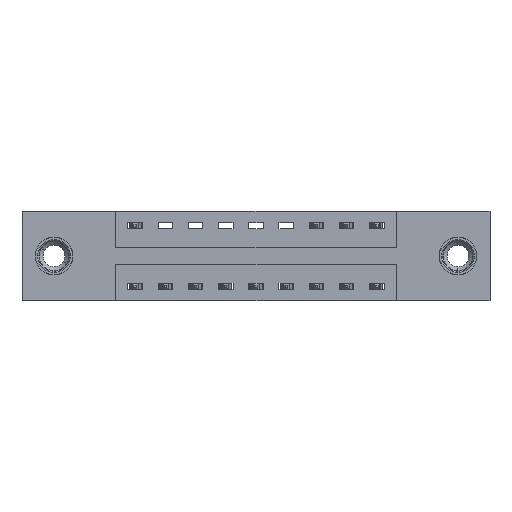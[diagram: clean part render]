
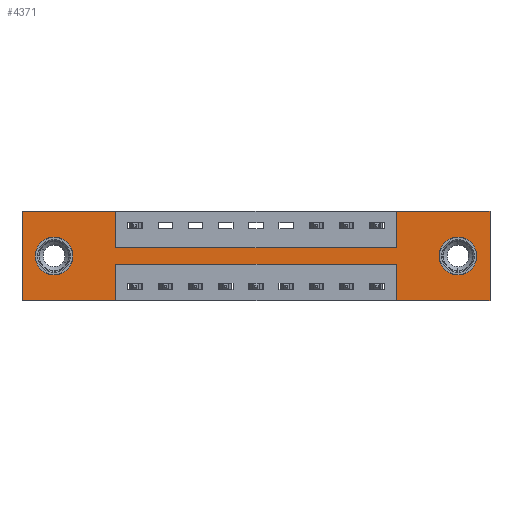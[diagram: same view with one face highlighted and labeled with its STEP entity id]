
A CAD part, front view. The second image highlights one B-rep face of the part: STEP entity #4371.
In plain terms, the highlighted planar face has unit normal (0, -1, 0).
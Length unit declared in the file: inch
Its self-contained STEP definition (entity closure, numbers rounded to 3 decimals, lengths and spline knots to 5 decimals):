
#75 = LINE ( 'NONE', #1002, #4664 ) ;
#83 = ORIENTED_EDGE ( 'NONE', *, *, #7281, .T. ) ;
#263 = DIRECTION ( 'NONE',  ( 0., 0., -1. ) ) ;
#331 = EDGE_CURVE ( 'NONE', #4508, #7372, #1394, .T. ) ;
#455 = EDGE_CURVE ( 'NONE', #640, #3458, #11091, .T. ) ;
#507 = LINE ( 'NONE', #1599, #2647 ) ;
#540 = CARTESIAN_POINT ( 'NONE',  ( 1.935, 0., 0. ) ) ;
#574 = LINE ( 'NONE', #8407, #2717 ) ;
#582 = VECTOR ( 'NONE', #7790, 39.37008 ) ;
#640 = VERTEX_POINT ( 'NONE', #8382 ) ;
#644 = DIRECTION ( 'NONE',  ( 0., 1., 0. ) ) ;
#896 = DIRECTION ( 'NONE',  ( 0., 0., -1. ) ) ;
#901 = CARTESIAN_POINT ( 'NONE',  ( 1.8025, 0., -0.263 ) ) ;
#913 = DIRECTION ( 'NONE',  ( 0., 0., 1. ) ) ;
#1002 = CARTESIAN_POINT ( 'NONE',  ( 0., 0., 0. ) ) ;
#1138 = EDGE_CURVE ( 'NONE', #10862, #8465, #2235, .T. ) ;
#1222 = DIRECTION ( 'NONE',  ( -1., 0., 0. ) ) ;
#1394 = LINE ( 'NONE', #3460, #9942 ) ;
#1597 = CARTESIAN_POINT ( 'NONE',  ( 0.3875, 0., -0.15 ) ) ;
#1599 = CARTESIAN_POINT ( 'NONE',  ( 0., 0., 0. ) ) ;
#1640 = LINE ( 'NONE', #8945, #6223 ) ;
#1676 = EDGE_CURVE ( 'NONE', #3062, #5204, #8653, .T. ) ;
#1693 = DIRECTION ( 'NONE',  ( 0., 0., 1. ) ) ;
#1708 = DIRECTION ( 'NONE',  ( 0., 1., 0. ) ) ;
#1754 = ORIENTED_EDGE ( 'NONE', *, *, #9610, .F. ) ;
#1829 = EDGE_CURVE ( 'NONE', #5204, #2667, #75, .T. ) ;
#1841 = ORIENTED_EDGE ( 'NONE', *, *, #1676, .F. ) ;
#1868 = DIRECTION ( 'NONE',  ( -1., 0., 0. ) ) ;
#1909 = AXIS2_PLACEMENT_3D ( 'NONE', #10047, #10891, #5828 ) ;
#2031 = FACE_BOUND ( 'NONE', #7180, .T. ) ;
#2183 = VECTOR ( 'NONE', #10526, 39.37008 ) ;
#2235 = CIRCLE ( 'NONE', #2948, 0.078 ) ;
#2348 = ORIENTED_EDGE ( 'NONE', *, *, #2852, .T. ) ;
#2382 = CARTESIAN_POINT ( 'NONE',  ( 0.3875, 0., -0.22 ) ) ;
#2465 = CARTESIAN_POINT ( 'NONE',  ( 0.1325, 0., -0.263 ) ) ;
#2504 = DIRECTION ( 'NONE',  ( 0., 0., 1. ) ) ;
#2592 = CARTESIAN_POINT ( 'NONE',  ( 1.5475, 0., 0. ) ) ;
#2647 = VECTOR ( 'NONE', #2504, 39.37008 ) ;
#2667 = VERTEX_POINT ( 'NONE', #540 ) ;
#2676 = EDGE_LOOP ( 'NONE', ( #4626, #8296, #4585, #8202, #4001, #7275, #1841, #6324, #8950, #9766, #1754, #2783 ) ) ;
#2717 = VECTOR ( 'NONE', #1222, 39.37008 ) ;
#2737 = VECTOR ( 'NONE', #263, 39.37008 ) ;
#2783 = ORIENTED_EDGE ( 'NONE', *, *, #7075, .F. ) ;
#2852 = EDGE_CURVE ( 'NONE', #8465, #10862, #10680, .T. ) ;
#2924 = EDGE_CURVE ( 'NONE', #6857, #3338, #9629, .T. ) ;
#2948 = AXIS2_PLACEMENT_3D ( 'NONE', #3736, #9827, #4658 ) ;
#3062 = VERTEX_POINT ( 'NONE', #8241 ) ;
#3338 = VERTEX_POINT ( 'NONE', #10388 ) ;
#3439 = VECTOR ( 'NONE', #8059, 39.37008 ) ;
#3458 = VERTEX_POINT ( 'NONE', #4564 ) ;
#3460 = CARTESIAN_POINT ( 'NONE',  ( 0.3875, 0., -0.37 ) ) ;
#3647 = ORIENTED_EDGE ( 'NONE', *, *, #1138, .T. ) ;
#3736 = CARTESIAN_POINT ( 'NONE',  ( 0.1325, 0., -0.185 ) ) ;
#3988 = PLANE ( 'NONE',  #1909 ) ;
#4001 = ORIENTED_EDGE ( 'NONE', *, *, #6166, .F. ) ;
#4012 = VERTEX_POINT ( 'NONE', #1597 ) ;
#4122 = EDGE_CURVE ( 'NONE', #4012, #3062, #9483, .T. ) ;
#4233 = VECTOR ( 'NONE', #1693, 39.37008 ) ;
#4371 = ADVANCED_FACE ( 'NONE', ( #8854, #2031, #6901 ), #3988, .T. ) ;
#4398 = EDGE_LOOP ( 'NONE', ( #83, #4752 ) ) ;
#4501 = EDGE_CURVE ( 'NONE', #6883, #4508, #4889, .T. ) ;
#4508 = VERTEX_POINT ( 'NONE', #9427 ) ;
#4554 = DIRECTION ( 'NONE',  ( 1., 0., 0. ) ) ;
#4564 = CARTESIAN_POINT ( 'NONE',  ( 0.3875, 0., 0. ) ) ;
#4585 = ORIENTED_EDGE ( 'NONE', *, *, #8102, .F. ) ;
#4626 = ORIENTED_EDGE ( 'NONE', *, *, #331, .F. ) ;
#4658 = DIRECTION ( 'NONE',  ( 0., 0., 1. ) ) ;
#4664 = VECTOR ( 'NONE', #9811, 39.37008 ) ;
#4752 = ORIENTED_EDGE ( 'NONE', *, *, #2924, .T. ) ;
#4889 = LINE ( 'NONE', #2382, #582 ) ;
#5204 = VERTEX_POINT ( 'NONE', #6087 ) ;
#5256 = VERTEX_POINT ( 'NONE', #11174 ) ;
#5293 = CIRCLE ( 'NONE', #5367, 0.078 ) ;
#5367 = AXIS2_PLACEMENT_3D ( 'NONE', #6141, #644, #7060 ) ;
#5828 = DIRECTION ( 'NONE',  ( 0., 0., -1. ) ) ;
#6087 = CARTESIAN_POINT ( 'NONE',  ( 1.5475, 0., 0. ) ) ;
#6114 = AXIS2_PLACEMENT_3D ( 'NONE', #7177, #1708, #8020 ) ;
#6141 = CARTESIAN_POINT ( 'NONE',  ( 1.8025, 0., -0.185 ) ) ;
#6166 = EDGE_CURVE ( 'NONE', #2667, #7441, #9739, .T. ) ;
#6177 = CARTESIAN_POINT ( 'NONE',  ( 0.1325, 0., -0.107 ) ) ;
#6223 = VECTOR ( 'NONE', #1868, 39.37008 ) ;
#6242 = DIRECTION ( 'NONE',  ( 0., 0., -1. ) ) ;
#6324 = ORIENTED_EDGE ( 'NONE', *, *, #4122, .F. ) ;
#6389 = DIRECTION ( 'NONE',  ( 0., 1., 0. ) ) ;
#6669 = CARTESIAN_POINT ( 'NONE',  ( 1.935, 0., 0. ) ) ;
#6814 = EDGE_CURVE ( 'NONE', #3458, #4012, #8222, .T. ) ;
#6857 = VERTEX_POINT ( 'NONE', #901 ) ;
#6883 = VERTEX_POINT ( 'NONE', #10597 ) ;
#6901 = FACE_OUTER_BOUND ( 'NONE', #2676, .T. ) ;
#7060 = DIRECTION ( 'NONE',  ( 0., 0., -1. ) ) ;
#7075 = EDGE_CURVE ( 'NONE', #7372, #5256, #574, .T. ) ;
#7177 = CARTESIAN_POINT ( 'NONE',  ( 0.1325, 0., -0.185 ) ) ;
#7180 = EDGE_LOOP ( 'NONE', ( #3647, #2348 ) ) ;
#7242 = CARTESIAN_POINT ( 'NONE',  ( 1.935, 0., -0.37 ) ) ;
#7275 = ORIENTED_EDGE ( 'NONE', *, *, #1829, .F. ) ;
#7281 = EDGE_CURVE ( 'NONE', #3338, #6857, #5293, .T. ) ;
#7372 = VERTEX_POINT ( 'NONE', #10430 ) ;
#7441 = VERTEX_POINT ( 'NONE', #7242 ) ;
#7790 = DIRECTION ( 'NONE',  ( -1., 0., 0. ) ) ;
#7918 = LINE ( 'NONE', #8145, #10090 ) ;
#8020 = DIRECTION ( 'NONE',  ( 0., 0., 1. ) ) ;
#8059 = DIRECTION ( 'NONE',  ( 0., 0., -1. ) ) ;
#8102 = EDGE_CURVE ( 'NONE', #11102, #6883, #7918, .T. ) ;
#8145 = CARTESIAN_POINT ( 'NONE',  ( 1.5475, 0., -0.37 ) ) ;
#8202 = ORIENTED_EDGE ( 'NONE', *, *, #10376, .F. ) ;
#8222 = LINE ( 'NONE', #9638, #3439 ) ;
#8241 = CARTESIAN_POINT ( 'NONE',  ( 1.5475, 0., -0.15 ) ) ;
#8296 = ORIENTED_EDGE ( 'NONE', *, *, #4501, .F. ) ;
#8382 = CARTESIAN_POINT ( 'NONE',  ( 0., 0., 0. ) ) ;
#8407 = CARTESIAN_POINT ( 'NONE',  ( 0., 0., -0.37 ) ) ;
#8465 = VERTEX_POINT ( 'NONE', #2465 ) ;
#8653 = LINE ( 'NONE', #2592, #4233 ) ;
#8854 = FACE_BOUND ( 'NONE', #4398, .T. ) ;
#8921 = CARTESIAN_POINT ( 'NONE',  ( 0., 0., 0. ) ) ;
#8923 = VECTOR ( 'NONE', #4554, 39.37008 ) ;
#8945 = CARTESIAN_POINT ( 'NONE',  ( 0., 0., -0.37 ) ) ;
#8950 = ORIENTED_EDGE ( 'NONE', *, *, #6814, .F. ) ;
#9073 = CARTESIAN_POINT ( 'NONE',  ( 1.5475, 0., -0.37 ) ) ;
#9427 = CARTESIAN_POINT ( 'NONE',  ( 0.3875, 0., -0.22 ) ) ;
#9483 = LINE ( 'NONE', #9680, #2183 ) ;
#9503 = AXIS2_PLACEMENT_3D ( 'NONE', #11374, #6389, #896 ) ;
#9610 = EDGE_CURVE ( 'NONE', #5256, #640, #507, .T. ) ;
#9629 = CIRCLE ( 'NONE', #9503, 0.078 ) ;
#9638 = CARTESIAN_POINT ( 'NONE',  ( 0.3875, 0., 0. ) ) ;
#9680 = CARTESIAN_POINT ( 'NONE',  ( 0.3875, 0., -0.15 ) ) ;
#9739 = LINE ( 'NONE', #6669, #2737 ) ;
#9766 = ORIENTED_EDGE ( 'NONE', *, *, #455, .F. ) ;
#9811 = DIRECTION ( 'NONE',  ( 1., 0., 0. ) ) ;
#9827 = DIRECTION ( 'NONE',  ( 0., 1., 0. ) ) ;
#9942 = VECTOR ( 'NONE', #6242, 39.37008 ) ;
#10047 = CARTESIAN_POINT ( 'NONE',  ( 0., 0., -0.37 ) ) ;
#10090 = VECTOR ( 'NONE', #913, 39.37008 ) ;
#10376 = EDGE_CURVE ( 'NONE', #7441, #11102, #1640, .T. ) ;
#10388 = CARTESIAN_POINT ( 'NONE',  ( 1.8025, 0., -0.107 ) ) ;
#10430 = CARTESIAN_POINT ( 'NONE',  ( 0.3875, 0., -0.37 ) ) ;
#10526 = DIRECTION ( 'NONE',  ( 1., 0., 0. ) ) ;
#10597 = CARTESIAN_POINT ( 'NONE',  ( 1.5475, 0., -0.22 ) ) ;
#10680 = CIRCLE ( 'NONE', #6114, 0.078 ) ;
#10862 = VERTEX_POINT ( 'NONE', #6177 ) ;
#10891 = DIRECTION ( 'NONE',  ( 0., -1., 0. ) ) ;
#11091 = LINE ( 'NONE', #8921, #8923 ) ;
#11102 = VERTEX_POINT ( 'NONE', #9073 ) ;
#11174 = CARTESIAN_POINT ( 'NONE',  ( 0., 0., -0.37 ) ) ;
#11374 = CARTESIAN_POINT ( 'NONE',  ( 1.8025, 0., -0.185 ) ) ;
